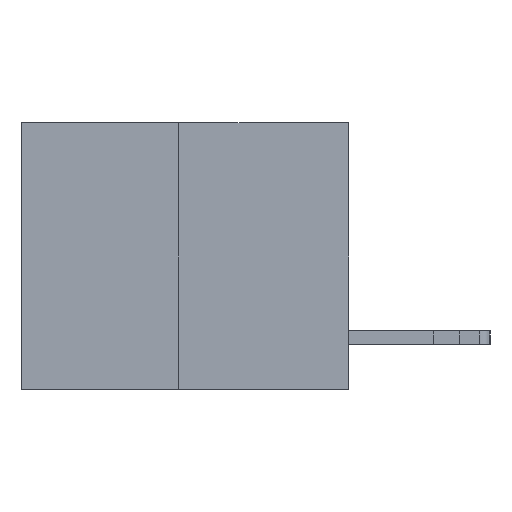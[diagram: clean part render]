
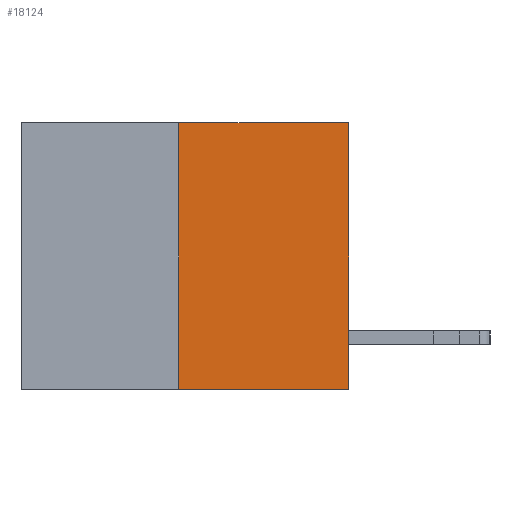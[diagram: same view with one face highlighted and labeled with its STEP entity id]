
A CAD part, left-side view. The second image highlights one B-rep face of the part: STEP entity #18124.
In plain terms, the highlighted planar face has unit normal (-1, 0, 0).
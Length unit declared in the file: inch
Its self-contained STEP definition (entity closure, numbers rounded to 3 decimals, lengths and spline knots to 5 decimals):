
#778 = ORIENTED_EDGE ( 'NONE', *, *, #14750, .T. ) ;
#2014 = EDGE_LOOP ( 'NONE', ( #3733, #5637, #778, #2788 ) ) ;
#2788 = ORIENTED_EDGE ( 'NONE', *, *, #7614, .F. ) ;
#3068 = EDGE_CURVE ( 'NONE', #5906, #4587, #11415, .T. ) ;
#3733 = ORIENTED_EDGE ( 'NONE', *, *, #15604, .F. ) ;
#3804 = FACE_OUTER_BOUND ( 'NONE', #2014, .T. ) ;
#4363 = CARTESIAN_POINT ( 'NONE',  ( 0., 0., -0.49 ) ) ;
#4587 = VERTEX_POINT ( 'NONE', #4363 ) ;
#4672 = AXIS2_PLACEMENT_3D ( 'NONE', #8918, #10711, #15853 ) ;
#5324 = PLANE ( 'NONE',  #4672 ) ;
#5369 = CARTESIAN_POINT ( 'NONE',  ( 0., 0.312, -0.49 ) ) ;
#5519 = LINE ( 'NONE', #5369, #8238 ) ;
#5637 = ORIENTED_EDGE ( 'NONE', *, *, #3068, .T. ) ;
#5906 = VERTEX_POINT ( 'NONE', #16751 ) ;
#6413 = CARTESIAN_POINT ( 'NONE',  ( 0., 0.312, 0. ) ) ;
#6832 = VECTOR ( 'NONE', #20211, 39.37008 ) ;
#7614 = EDGE_CURVE ( 'NONE', #12482, #22773, #12410, .T. ) ;
#7964 = VECTOR ( 'NONE', #14853, 39.37008 ) ;
#8238 = VECTOR ( 'NONE', #20971, 39.37008 ) ;
#8918 = CARTESIAN_POINT ( 'NONE',  ( 0., 0.6, 0. ) ) ;
#9259 = DIRECTION ( 'NONE',  ( 0., -1., 0. ) ) ;
#10284 = VECTOR ( 'NONE', #9259, 39.37008 ) ;
#10711 = DIRECTION ( 'NONE',  ( 1., 0., 0. ) ) ;
#11361 = CARTESIAN_POINT ( 'NONE',  ( 0., 0.6, 0. ) ) ;
#11415 = LINE ( 'NONE', #21807, #10284 ) ;
#12410 = LINE ( 'NONE', #11361, #6832 ) ;
#12482 = VERTEX_POINT ( 'NONE', #6413 ) ;
#14750 = EDGE_CURVE ( 'NONE', #4587, #22773, #16892, .T. ) ;
#14853 = DIRECTION ( 'NONE',  ( 0., 0., 1. ) ) ;
#15604 = EDGE_CURVE ( 'NONE', #5906, #12482, #5519, .T. ) ;
#15853 = DIRECTION ( 'NONE',  ( 0., 0., -1. ) ) ;
#16751 = CARTESIAN_POINT ( 'NONE',  ( 0., 0.312, -0.49 ) ) ;
#16892 = LINE ( 'NONE', #20114, #7964 ) ;
#18124 = ADVANCED_FACE ( 'NONE', ( #3804 ), #5324, .F. ) ;
#20114 = CARTESIAN_POINT ( 'NONE',  ( 0., 0., 0. ) ) ;
#20211 = DIRECTION ( 'NONE',  ( 0., -1., 0. ) ) ;
#20971 = DIRECTION ( 'NONE',  ( 0., 0., 1. ) ) ;
#21634 = CARTESIAN_POINT ( 'NONE',  ( 0., 0., 0. ) ) ;
#21807 = CARTESIAN_POINT ( 'NONE',  ( 0., 0.6, -0.49 ) ) ;
#22773 = VERTEX_POINT ( 'NONE', #21634 ) ;
